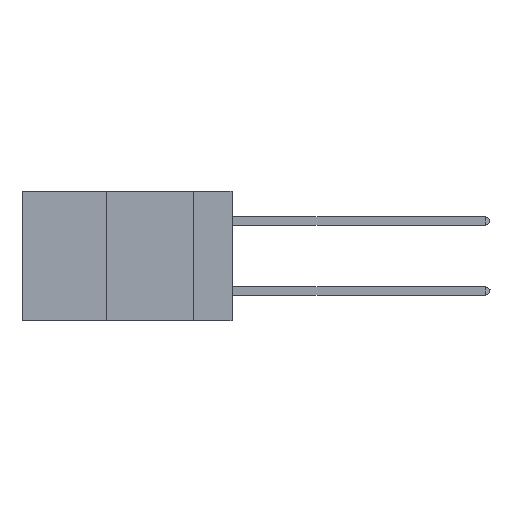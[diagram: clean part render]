
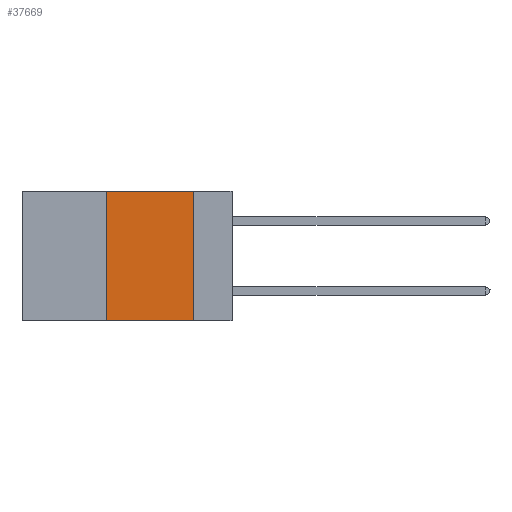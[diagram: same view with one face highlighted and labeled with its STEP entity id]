
A CAD part, left-side view. The second image highlights one B-rep face of the part: STEP entity #37669.
In plain terms, the highlighted planar face has unit normal (-1, 0, 0).
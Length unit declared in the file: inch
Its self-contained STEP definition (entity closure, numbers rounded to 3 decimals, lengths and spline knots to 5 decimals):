
#1626 = DIRECTION ( 'NONE',  ( 0., 0., 1. ) ) ;
#3321 = ORIENTED_EDGE ( 'NONE', *, *, #26063, .F. ) ;
#5026 = VERTEX_POINT ( 'NONE', #38036 ) ;
#7748 = LINE ( 'NONE', #32474, #33494 ) ;
#8282 = DIRECTION ( 'NONE',  ( 1., 0., 0. ) ) ;
#9302 = ORIENTED_EDGE ( 'NONE', *, *, #19596, .F. ) ;
#11519 = PLANE ( 'NONE',  #15571 ) ;
#13091 = VECTOR ( 'NONE', #42471, 39.37008 ) ;
#15571 = AXIS2_PLACEMENT_3D ( 'NONE', #28408, #8282, #38669 ) ;
#16062 = LINE ( 'NONE', #19251, #28702 ) ;
#16726 = LINE ( 'NONE', #42767, #13091 ) ;
#16767 = VECTOR ( 'NONE', #1626, 39.37008 ) ;
#18625 = FACE_OUTER_BOUND ( 'NONE', #32642, .T. ) ;
#19251 = CARTESIAN_POINT ( 'NONE',  ( 0., 0.6, 0. ) ) ;
#19596 = EDGE_CURVE ( 'NONE', #41426, #28959, #16062, .T. ) ;
#26063 = EDGE_CURVE ( 'NONE', #40206, #41426, #33075, .T. ) ;
#26221 = EDGE_CURVE ( 'NONE', #28959, #5026, #16726, .T. ) ;
#28408 = CARTESIAN_POINT ( 'NONE',  ( 0., 0.6, 0. ) ) ;
#28702 = VECTOR ( 'NONE', #42743, 39.37008 ) ;
#28959 = VERTEX_POINT ( 'NONE', #39483 ) ;
#31144 = CARTESIAN_POINT ( 'NONE',  ( 0., 0.36, 0. ) ) ;
#31912 = DIRECTION ( 'NONE',  ( 0., -1., 0. ) ) ;
#32474 = CARTESIAN_POINT ( 'NONE',  ( 0., 0.6, -0.37 ) ) ;
#32642 = EDGE_LOOP ( 'NONE', ( #35551, #9302, #3321, #41269 ) ) ;
#33075 = LINE ( 'NONE', #38791, #16767 ) ;
#33494 = VECTOR ( 'NONE', #31912, 39.37008 ) ;
#35551 = ORIENTED_EDGE ( 'NONE', *, *, #26221, .F. ) ;
#37669 = ADVANCED_FACE ( 'NONE', ( #18625 ), #11519, .F. ) ;
#38036 = CARTESIAN_POINT ( 'NONE',  ( 0., 0.11, -0.37 ) ) ;
#38206 = CARTESIAN_POINT ( 'NONE',  ( 0., 0.36, -0.37 ) ) ;
#38669 = DIRECTION ( 'NONE',  ( 0., 0., -1. ) ) ;
#38791 = CARTESIAN_POINT ( 'NONE',  ( 0., 0.36, 0. ) ) ;
#39483 = CARTESIAN_POINT ( 'NONE',  ( 0., 0.11, 0. ) ) ;
#40206 = VERTEX_POINT ( 'NONE', #38206 ) ;
#41269 = ORIENTED_EDGE ( 'NONE', *, *, #42889, .T. ) ;
#41426 = VERTEX_POINT ( 'NONE', #31144 ) ;
#42471 = DIRECTION ( 'NONE',  ( 0., 0., -1. ) ) ;
#42743 = DIRECTION ( 'NONE',  ( 0., -1., 0. ) ) ;
#42767 = CARTESIAN_POINT ( 'NONE',  ( 0., 0.11, 0. ) ) ;
#42889 = EDGE_CURVE ( 'NONE', #40206, #5026, #7748, .T. ) ;
